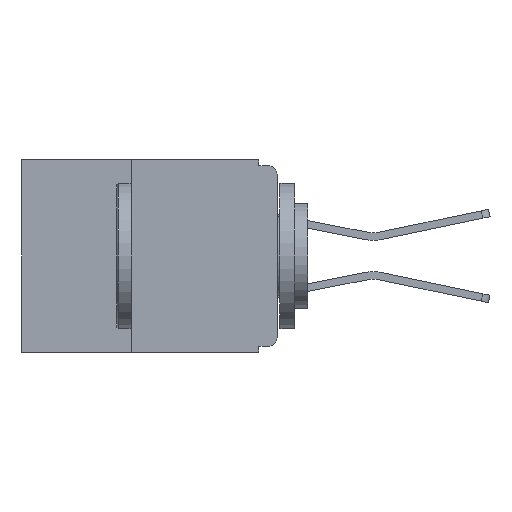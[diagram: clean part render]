
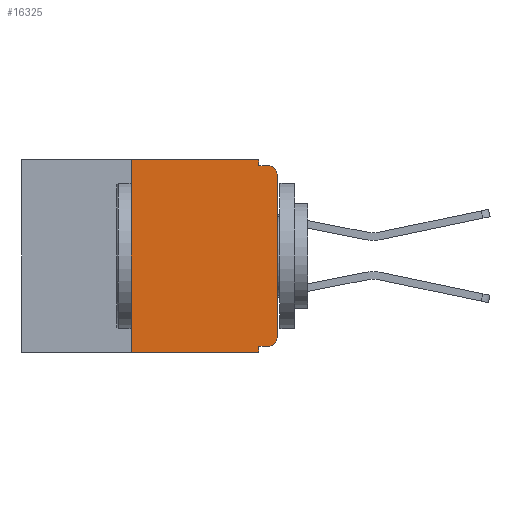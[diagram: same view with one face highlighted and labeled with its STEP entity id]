
A CAD part, left-side view. The second image highlights one B-rep face of the part: STEP entity #16325.
In plain terms, the highlighted planar face has unit normal (-1, 0, 0).
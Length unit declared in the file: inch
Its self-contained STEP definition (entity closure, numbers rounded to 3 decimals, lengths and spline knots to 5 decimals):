
#277 = LINE ( 'NONE', #5997, #4916 ) ;
#483 = LINE ( 'NONE', #8481, #10292 ) ;
#548 = ORIENTED_EDGE ( 'NONE', *, *, #2258, .T. ) ;
#1045 = CARTESIAN_POINT ( 'NONE',  ( 0., 0., -0.305 ) ) ;
#1524 = DIRECTION ( 'NONE',  ( 0., 0., 1. ) ) ;
#2258 = EDGE_CURVE ( 'NONE', #20358, #13486, #18861, .T. ) ;
#2288 = CARTESIAN_POINT ( 'NONE',  ( 0., 0.437, 0. ) ) ;
#2392 = ORIENTED_EDGE ( 'NONE', *, *, #3104, .F. ) ;
#2421 = EDGE_CURVE ( 'NONE', #13231, #7371, #277, .T. ) ;
#2441 = DIRECTION ( 'NONE',  ( 0., -1., 0. ) ) ;
#2485 = EDGE_CURVE ( 'NONE', #20358, #21831, #14036, .T. ) ;
#2944 = CARTESIAN_POINT ( 'NONE',  ( 0., 0.031, 0. ) ) ;
#3035 = LINE ( 'NONE', #16008, #3660 ) ;
#3104 = EDGE_CURVE ( 'NONE', #7922, #19412, #6399, .T. ) ;
#3660 = VECTOR ( 'NONE', #2441, 39.37008 ) ;
#3994 = AXIS2_PLACEMENT_3D ( 'NONE', #19181, #20544, #15750 ) ;
#4718 = LINE ( 'NONE', #20616, #19540 ) ;
#4779 = CARTESIAN_POINT ( 'NONE',  ( 0., 0., -0.32 ) ) ;
#4830 = CARTESIAN_POINT ( 'NONE',  ( 0., 0.031, -0.32 ) ) ;
#4916 = VECTOR ( 'NONE', #9687, 39.37008 ) ;
#5069 = EDGE_CURVE ( 'NONE', #7922, #7985, #483, .T. ) ;
#5227 = DIRECTION ( 'NONE',  ( 0., 0., -1. ) ) ;
#5254 = DIRECTION ( 'NONE',  ( -1., 0., 0. ) ) ;
#5260 = CARTESIAN_POINT ( 'NONE',  ( 0., 0.015, -0.025 ) ) ;
#5342 = EDGE_CURVE ( 'NONE', #9498, #6747, #20207, .T. ) ;
#5435 = ORIENTED_EDGE ( 'NONE', *, *, #2421, .F. ) ;
#5997 = CARTESIAN_POINT ( 'NONE',  ( 0., 0.031, 0. ) ) ;
#6399 = LINE ( 'NONE', #18625, #10369 ) ;
#6574 = AXIS2_PLACEMENT_3D ( 'NONE', #2288, #23343, #11843 ) ;
#6630 = EDGE_CURVE ( 'NONE', #7371, #6747, #4718, .T. ) ;
#6747 = VERTEX_POINT ( 'NONE', #15795 ) ;
#7353 = LINE ( 'NONE', #11292, #11329 ) ;
#7371 = VERTEX_POINT ( 'NONE', #20471 ) ;
#7922 = VERTEX_POINT ( 'NONE', #20201 ) ;
#7985 = VERTEX_POINT ( 'NONE', #19229 ) ;
#8151 = ORIENTED_EDGE ( 'NONE', *, *, #5342, .T. ) ;
#8444 = DIRECTION ( 'NONE',  ( 0., -1., 0. ) ) ;
#8481 = CARTESIAN_POINT ( 'NONE',  ( 0., 0.437, -0.33 ) ) ;
#8496 = ORIENTED_EDGE ( 'NONE', *, *, #21702, .F. ) ;
#9498 = VERTEX_POINT ( 'NONE', #13561 ) ;
#9680 = EDGE_CURVE ( 'NONE', #21831, #7985, #7353, .T. ) ;
#9687 = DIRECTION ( 'NONE',  ( 0., 0., -1. ) ) ;
#10009 = ORIENTED_EDGE ( 'NONE', *, *, #6630, .F. ) ;
#10075 = PLANE ( 'NONE',  #6574 ) ;
#10292 = VECTOR ( 'NONE', #8444, 39.37008 ) ;
#10369 = VECTOR ( 'NONE', #18511, 39.37008 ) ;
#10664 = CARTESIAN_POINT ( 'NONE',  ( 0., 0.25, 0. ) ) ;
#11201 = DIRECTION ( 'NONE',  ( 0., 0., -1. ) ) ;
#11292 = CARTESIAN_POINT ( 'NONE',  ( 0., 0.031, -0.33 ) ) ;
#11329 = VECTOR ( 'NONE', #11201, 39.37008 ) ;
#11501 = ORIENTED_EDGE ( 'NONE', *, *, #14807, .T. ) ;
#11843 = DIRECTION ( 'NONE',  ( 0., 0., -1. ) ) ;
#12466 = EDGE_LOOP ( 'NONE', ( #11501, #8151, #10009, #5435, #8496, #2392, #19086, #16974, #14282, #548 ) ) ;
#13231 = VERTEX_POINT ( 'NONE', #2944 ) ;
#13394 = VECTOR ( 'NONE', #1524, 39.37008 ) ;
#13486 = VERTEX_POINT ( 'NONE', #1045 ) ;
#13561 = CARTESIAN_POINT ( 'NONE',  ( 0., 0., -0.025 ) ) ;
#14036 = LINE ( 'NONE', #4779, #23634 ) ;
#14282 = ORIENTED_EDGE ( 'NONE', *, *, #2485, .F. ) ;
#14807 = EDGE_CURVE ( 'NONE', #13486, #9498, #18469, .T. ) ;
#15750 = DIRECTION ( 'NONE',  ( 0., 0., -1. ) ) ;
#15795 = CARTESIAN_POINT ( 'NONE',  ( 0., 0.015, -0.01 ) ) ;
#16008 = CARTESIAN_POINT ( 'NONE',  ( 0., 0.437, 0. ) ) ;
#16325 = ADVANCED_FACE ( 'NONE', ( #22577 ), #10075, .F. ) ;
#16974 = ORIENTED_EDGE ( 'NONE', *, *, #9680, .F. ) ;
#18469 = LINE ( 'NONE', #24691, #13394 ) ;
#18511 = DIRECTION ( 'NONE',  ( 0., 0., 1. ) ) ;
#18625 = CARTESIAN_POINT ( 'NONE',  ( 0., 0.25, -0.33 ) ) ;
#18861 = CIRCLE ( 'NONE', #3994, 0.015 ) ;
#19086 = ORIENTED_EDGE ( 'NONE', *, *, #5069, .T. ) ;
#19181 = CARTESIAN_POINT ( 'NONE',  ( 0., 0.015, -0.305 ) ) ;
#19229 = CARTESIAN_POINT ( 'NONE',  ( 0., 0.031, -0.33 ) ) ;
#19412 = VERTEX_POINT ( 'NONE', #10664 ) ;
#19540 = VECTOR ( 'NONE', #20489, 39.37008 ) ;
#20201 = CARTESIAN_POINT ( 'NONE',  ( 0., 0.25, -0.33 ) ) ;
#20207 = CIRCLE ( 'NONE', #21223, 0.015 ) ;
#20358 = VERTEX_POINT ( 'NONE', #21620 ) ;
#20471 = CARTESIAN_POINT ( 'NONE',  ( 0., 0.031, -0.01 ) ) ;
#20489 = DIRECTION ( 'NONE',  ( 0., -1., 0. ) ) ;
#20544 = DIRECTION ( 'NONE',  ( -1., 0., 0. ) ) ;
#20616 = CARTESIAN_POINT ( 'NONE',  ( 0., 0., -0.01 ) ) ;
#21223 = AXIS2_PLACEMENT_3D ( 'NONE', #5260, #5254, #5227 ) ;
#21620 = CARTESIAN_POINT ( 'NONE',  ( 0., 0.015, -0.32 ) ) ;
#21702 = EDGE_CURVE ( 'NONE', #19412, #13231, #3035, .T. ) ;
#21831 = VERTEX_POINT ( 'NONE', #4830 ) ;
#22577 = FACE_OUTER_BOUND ( 'NONE', #12466, .T. ) ;
#23343 = DIRECTION ( 'NONE',  ( 1., 0., 0. ) ) ;
#23634 = VECTOR ( 'NONE', #23717, 39.37008 ) ;
#23717 = DIRECTION ( 'NONE',  ( 0., 1., 0. ) ) ;
#24691 = CARTESIAN_POINT ( 'NONE',  ( 0., 0., 0. ) ) ;
